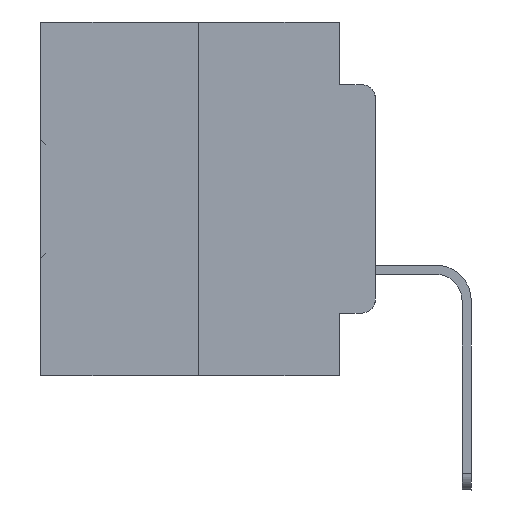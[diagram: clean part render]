
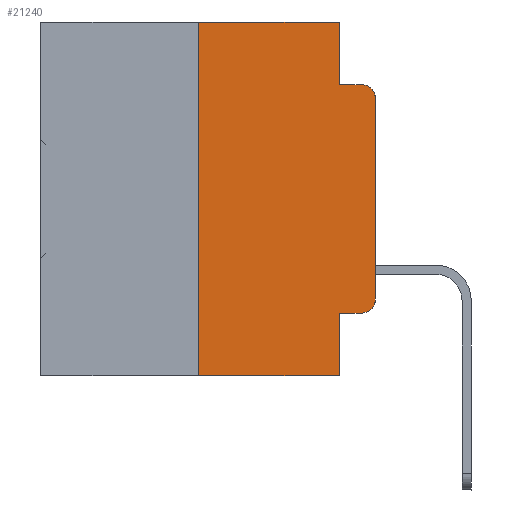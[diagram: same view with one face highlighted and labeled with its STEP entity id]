
A CAD part, left-side view. The second image highlights one B-rep face of the part: STEP entity #21240.
In plain terms, the highlighted planar face has unit normal (-1, 0, 0).
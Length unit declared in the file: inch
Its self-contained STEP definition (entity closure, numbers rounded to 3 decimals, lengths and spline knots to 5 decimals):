
#447 = VECTOR ( 'NONE', #8789, 39.37008 ) ;
#1366 = LINE ( 'NONE', #13010, #3924 ) ;
#1889 = DIRECTION ( 'NONE',  ( -1., 0., 0. ) ) ;
#2184 = LINE ( 'NONE', #18114, #29375 ) ;
#2268 = VERTEX_POINT ( 'NONE', #29627 ) ;
#3089 = VERTEX_POINT ( 'NONE', #3923 ) ;
#3322 = VECTOR ( 'NONE', #15926, 39.37008 ) ;
#3364 = ORIENTED_EDGE ( 'NONE', *, *, #20653, .T. ) ;
#3791 = VECTOR ( 'NONE', #29460, 39.37008 ) ;
#3923 = CARTESIAN_POINT ( 'NONE',  ( 0., 0., -0.3915 ) ) ;
#3924 = VECTOR ( 'NONE', #34568, 39.37008 ) ;
#4621 = ORIENTED_EDGE ( 'NONE', *, *, #9352, .F. ) ;
#4737 = DIRECTION ( 'NONE',  ( 0., 0., -1. ) ) ;
#5106 = CARTESIAN_POINT ( 'NONE',  ( 0., 0.051, -0.4115 ) ) ;
#5430 = EDGE_LOOP ( 'NONE', ( #32673, #3364, #6186, #4621, #29750, #7354, #28309, #27273, #31912, #14825 ) ) ;
#5939 = VERTEX_POINT ( 'NONE', #6963 ) ;
#6186 = ORIENTED_EDGE ( 'NONE', *, *, #31526, .F. ) ;
#6963 = CARTESIAN_POINT ( 'NONE',  ( 0., 0.051, -0.0885 ) ) ;
#7182 = VERTEX_POINT ( 'NONE', #12475 ) ;
#7354 = ORIENTED_EDGE ( 'NONE', *, *, #33622, .F. ) ;
#7413 = CIRCLE ( 'NONE', #7884, 0.02 ) ;
#7475 = DIRECTION ( 'NONE',  ( 1., 0., 0. ) ) ;
#7679 = AXIS2_PLACEMENT_3D ( 'NONE', #31305, #7475, #25947 ) ;
#7819 = EDGE_CURVE ( 'NONE', #7182, #16956, #14705, .T. ) ;
#7884 = AXIS2_PLACEMENT_3D ( 'NONE', #9755, #1889, #4737 ) ;
#8789 = DIRECTION ( 'NONE',  ( 0., 0., -1. ) ) ;
#9352 = EDGE_CURVE ( 'NONE', #16144, #5939, #1366, .T. ) ;
#9622 = CARTESIAN_POINT ( 'NONE',  ( 0., 0.25, 0. ) ) ;
#9657 = CIRCLE ( 'NONE', #26640, 0.02 ) ;
#9755 = CARTESIAN_POINT ( 'NONE',  ( 0., 0.02, -0.1085 ) ) ;
#11103 = EDGE_CURVE ( 'NONE', #3089, #21231, #30539, .T. ) ;
#11161 = LINE ( 'NONE', #29839, #27468 ) ;
#12475 = CARTESIAN_POINT ( 'NONE',  ( 0., 0.051, -0.4115 ) ) ;
#12774 = DIRECTION ( 'NONE',  ( -1., 0., 0. ) ) ;
#13010 = CARTESIAN_POINT ( 'NONE',  ( 0., 0.051, 0. ) ) ;
#13688 = CARTESIAN_POINT ( 'NONE',  ( 0., 0.051, 0. ) ) ;
#14705 = LINE ( 'NONE', #24352, #447 ) ;
#14825 = ORIENTED_EDGE ( 'NONE', *, *, #26813, .T. ) ;
#15244 = DIRECTION ( 'NONE',  ( 0., 0., -1. ) ) ;
#15926 = DIRECTION ( 'NONE',  ( 0., -1., 0. ) ) ;
#16144 = VERTEX_POINT ( 'NONE', #13688 ) ;
#16956 = VERTEX_POINT ( 'NONE', #30859 ) ;
#17532 = LINE ( 'NONE', #23854, #3322 ) ;
#17774 = EDGE_CURVE ( 'NONE', #7182, #21518, #26480, .T. ) ;
#17908 = CARTESIAN_POINT ( 'NONE',  ( 0., 0., -0.1085 ) ) ;
#18114 = CARTESIAN_POINT ( 'NONE',  ( 0., 0.051, -0.0885 ) ) ;
#18697 = DIRECTION ( 'NONE',  ( 0., 0., 1. ) ) ;
#19111 = DIRECTION ( 'NONE',  ( 0., -1., 0. ) ) ;
#20497 = FACE_OUTER_BOUND ( 'NONE', #5430, .T. ) ;
#20653 = EDGE_CURVE ( 'NONE', #21231, #30516, #7413, .T. ) ;
#21022 = VECTOR ( 'NONE', #34613, 39.37008 ) ;
#21231 = VERTEX_POINT ( 'NONE', #17908 ) ;
#21240 = ADVANCED_FACE ( 'NONE', ( #20497 ), #28621, .F. ) ;
#21518 = VERTEX_POINT ( 'NONE', #30022 ) ;
#23854 = CARTESIAN_POINT ( 'NONE',  ( 0., 0.473, 0. ) ) ;
#24098 = CARTESIAN_POINT ( 'NONE',  ( 0., 0., 0. ) ) ;
#24196 = CARTESIAN_POINT ( 'NONE',  ( 0., 0.25, 0. ) ) ;
#24352 = CARTESIAN_POINT ( 'NONE',  ( 0., 0.051, 0. ) ) ;
#25863 = CARTESIAN_POINT ( 'NONE',  ( 0., 0.02, -0.3915 ) ) ;
#25947 = DIRECTION ( 'NONE',  ( 0., 0., -1. ) ) ;
#26480 = LINE ( 'NONE', #5106, #21022 ) ;
#26640 = AXIS2_PLACEMENT_3D ( 'NONE', #25863, #12774, #15244 ) ;
#26739 = VERTEX_POINT ( 'NONE', #9622 ) ;
#26813 = EDGE_CURVE ( 'NONE', #21518, #3089, #9657, .T. ) ;
#27273 = ORIENTED_EDGE ( 'NONE', *, *, #7819, .F. ) ;
#27468 = VECTOR ( 'NONE', #19111, 39.37008 ) ;
#27520 = EDGE_CURVE ( 'NONE', #26739, #16144, #17532, .T. ) ;
#28309 = ORIENTED_EDGE ( 'NONE', *, *, #29224, .T. ) ;
#28487 = DIRECTION ( 'NONE',  ( 0., -1., 0. ) ) ;
#28621 = PLANE ( 'NONE',  #7679 ) ;
#29224 = EDGE_CURVE ( 'NONE', #2268, #16956, #11161, .T. ) ;
#29375 = VECTOR ( 'NONE', #28487, 39.37008 ) ;
#29460 = DIRECTION ( 'NONE',  ( 0., 0., 1. ) ) ;
#29627 = CARTESIAN_POINT ( 'NONE',  ( 0., 0.25, -0.5 ) ) ;
#29750 = ORIENTED_EDGE ( 'NONE', *, *, #27520, .F. ) ;
#29839 = CARTESIAN_POINT ( 'NONE',  ( 0., 0.473, -0.5 ) ) ;
#30022 = CARTESIAN_POINT ( 'NONE',  ( 0., 0.02, -0.4115 ) ) ;
#30516 = VERTEX_POINT ( 'NONE', #32863 ) ;
#30539 = LINE ( 'NONE', #24098, #3791 ) ;
#30859 = CARTESIAN_POINT ( 'NONE',  ( 0., 0.051, -0.5 ) ) ;
#31211 = LINE ( 'NONE', #24196, #32065 ) ;
#31305 = CARTESIAN_POINT ( 'NONE',  ( 0., 0.473, 0. ) ) ;
#31526 = EDGE_CURVE ( 'NONE', #5939, #30516, #2184, .T. ) ;
#31912 = ORIENTED_EDGE ( 'NONE', *, *, #17774, .T. ) ;
#32065 = VECTOR ( 'NONE', #18697, 39.37008 ) ;
#32673 = ORIENTED_EDGE ( 'NONE', *, *, #11103, .T. ) ;
#32863 = CARTESIAN_POINT ( 'NONE',  ( 0., 0.02, -0.0885 ) ) ;
#33622 = EDGE_CURVE ( 'NONE', #2268, #26739, #31211, .T. ) ;
#34568 = DIRECTION ( 'NONE',  ( 0., 0., -1. ) ) ;
#34613 = DIRECTION ( 'NONE',  ( 0., -1., 0. ) ) ;
